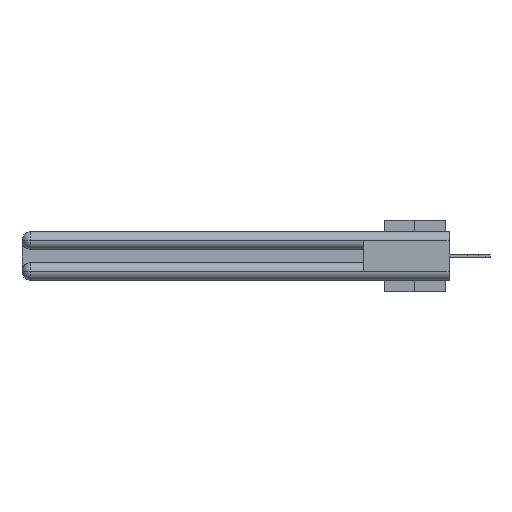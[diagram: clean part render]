
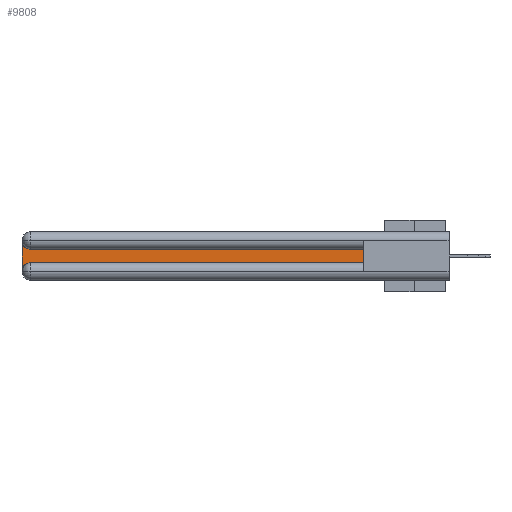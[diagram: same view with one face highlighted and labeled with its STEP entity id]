
A CAD part, left-side view. The second image highlights one B-rep face of the part: STEP entity #9808.
In plain terms, the highlighted planar face has unit normal (-1, 0, 0).
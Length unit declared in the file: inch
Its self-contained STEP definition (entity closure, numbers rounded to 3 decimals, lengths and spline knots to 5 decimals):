
#23 = EDGE_LOOP ( 'NONE', ( #13880, #32279, #25327, #1078, #20939, #4430 ) ) ;
#69 = CIRCLE ( 'NONE', #11544, 0.06 ) ;
#161 = CARTESIAN_POINT ( 'NONE',  ( 0.075, 2.94, -0.2175 ) ) ;
#1078 = ORIENTED_EDGE ( 'NONE', *, *, #13162, .T. ) ;
#3026 = EDGE_CURVE ( 'NONE', #12089, #25426, #20603, .T. ) ;
#4104 = EDGE_CURVE ( 'NONE', #23388, #17928, #10779, .T. ) ;
#4430 = ORIENTED_EDGE ( 'NONE', *, *, #17665, .T. ) ;
#5667 = DIRECTION ( 'NONE',  ( 0., 0., 1. ) ) ;
#6510 = CARTESIAN_POINT ( 'NONE',  ( 0.075, 3., -0.0625 ) ) ;
#6605 = CARTESIAN_POINT ( 'NONE',  ( 0.075, 0.6, -0.1225 ) ) ;
#7577 = DIRECTION ( 'NONE',  ( 1., 0., 0. ) ) ;
#8205 = CARTESIAN_POINT ( 'NONE',  ( 0.075, 3., -0.1225 ) ) ;
#8288 = CARTESIAN_POINT ( 'NONE',  ( 0.075, 2.94, -0.0625 ) ) ;
#9515 = VERTEX_POINT ( 'NONE', #13134 ) ;
#9808 = ADVANCED_FACE ( 'NONE', ( #32837 ), #17015, .F. ) ;
#10272 = LINE ( 'NONE', #21615, #35126 ) ;
#10779 = LINE ( 'NONE', #27175, #21799 ) ;
#11139 = DIRECTION ( 'NONE',  ( 0., -1., 0. ) ) ;
#11151 = AXIS2_PLACEMENT_3D ( 'NONE', #8205, #19186, #17195 ) ;
#11246 = LINE ( 'NONE', #30126, #15208 ) ;
#11544 = AXIS2_PLACEMENT_3D ( 'NONE', #13327, #7577, #29854 ) ;
#12089 = VERTEX_POINT ( 'NONE', #25118 ) ;
#13134 = CARTESIAN_POINT ( 'NONE',  ( 0.075, 3., -0.2775 ) ) ;
#13162 = EDGE_CURVE ( 'NONE', #9515, #23388, #69, .T. ) ;
#13327 = CARTESIAN_POINT ( 'NONE',  ( 0.075, 2.94, -0.2775 ) ) ;
#13880 = ORIENTED_EDGE ( 'NONE', *, *, #3026, .T. ) ;
#15208 = VECTOR ( 'NONE', #5667, 39.37008 ) ;
#17015 = PLANE ( 'NONE',  #11151 ) ;
#17104 = DIRECTION ( 'NONE',  ( 0., 0., -1. ) ) ;
#17195 = DIRECTION ( 'NONE',  ( 0., 0., -1. ) ) ;
#17665 = EDGE_CURVE ( 'NONE', #17928, #12089, #11246, .T. ) ;
#17928 = VERTEX_POINT ( 'NONE', #19141 ) ;
#18334 = EDGE_CURVE ( 'NONE', #21024, #9515, #10272, .T. ) ;
#19141 = CARTESIAN_POINT ( 'NONE',  ( 0.075, 0.6, -0.2175 ) ) ;
#19186 = DIRECTION ( 'NONE',  ( 1., 0., 0. ) ) ;
#20603 = LINE ( 'NONE', #6605, #30904 ) ;
#20939 = ORIENTED_EDGE ( 'NONE', *, *, #4104, .T. ) ;
#21024 = VERTEX_POINT ( 'NONE', #6510 ) ;
#21615 = CARTESIAN_POINT ( 'NONE',  ( 0.075, 3., -0.2175 ) ) ;
#21799 = VECTOR ( 'NONE', #11139, 39.37008 ) ;
#22988 = EDGE_CURVE ( 'NONE', #25426, #21024, #28928, .T. ) ;
#23388 = VERTEX_POINT ( 'NONE', #161 ) ;
#23492 = DIRECTION ( 'NONE',  ( 0., 1., 0. ) ) ;
#25118 = CARTESIAN_POINT ( 'NONE',  ( 0.075, 0.6, -0.1225 ) ) ;
#25327 = ORIENTED_EDGE ( 'NONE', *, *, #18334, .T. ) ;
#25426 = VERTEX_POINT ( 'NONE', #30758 ) ;
#27175 = CARTESIAN_POINT ( 'NONE',  ( 0.075, 0.6, -0.2175 ) ) ;
#27527 = DIRECTION ( 'NONE',  ( 1., 0., 0. ) ) ;
#28928 = CIRCLE ( 'NONE', #34090, 0.06 ) ;
#29854 = DIRECTION ( 'NONE',  ( 0., 0., -1. ) ) ;
#29875 = DIRECTION ( 'NONE',  ( 0., 0., -1. ) ) ;
#30126 = CARTESIAN_POINT ( 'NONE',  ( 0.075, 0.6, -0.2175 ) ) ;
#30758 = CARTESIAN_POINT ( 'NONE',  ( 0.075, 2.94, -0.1225 ) ) ;
#30904 = VECTOR ( 'NONE', #23492, 39.37008 ) ;
#32279 = ORIENTED_EDGE ( 'NONE', *, *, #22988, .T. ) ;
#32837 = FACE_OUTER_BOUND ( 'NONE', #23, .T. ) ;
#34090 = AXIS2_PLACEMENT_3D ( 'NONE', #8288, #27527, #17104 ) ;
#35126 = VECTOR ( 'NONE', #29875, 39.37008 ) ;
